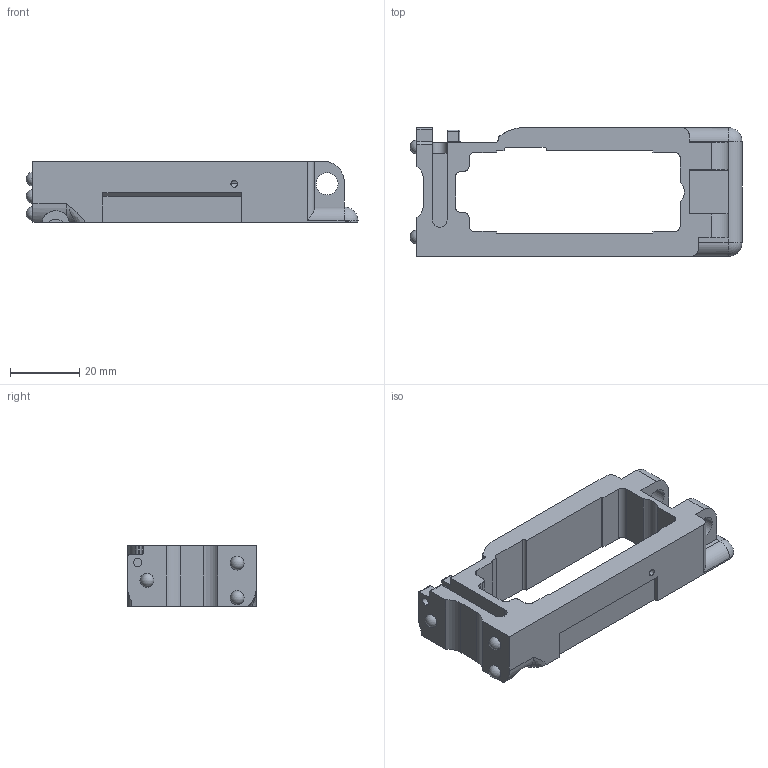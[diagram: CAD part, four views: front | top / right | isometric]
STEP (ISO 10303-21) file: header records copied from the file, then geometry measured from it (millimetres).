
FILE_DESCRIPTION (( 'STEP AP214' ), '1' );
FILE_NAME ('Magwell_1.STEP', '2013-09-01T16:47:27', ( 'Asher' ), ( '' ), 'SwSTEP 2.0', 'SolidWorks 2013', '' );
FILE_SCHEMA (( 'AUTOMOTIVE_DESIGN' ));
Length unit declared in the file: millimetre
Products named in the file (1): Magwell_1
Bounding box: 95.81 x 37.13 x 17.46 mm (x, y, z)
Volume: 24764.6 mm3; surface area: 12778.3 mm2
Topology: 1 solids, 1 shells, 151 faces, 454 edges, 295 vertices
Faces by surface type: plane 64, cylinder 61, sphere 20, cone 2, bspline 2, torus 2
Entity records: 5084 total; most frequent: CARTESIAN_POINT 1075, DIRECTION 845, ORIENTED_EDGE 826, EDGE_CURVE 413, AXIS2_PLACEMENT_3D 301, VERTEX_POINT 278, LINE 243, VECTOR 243
